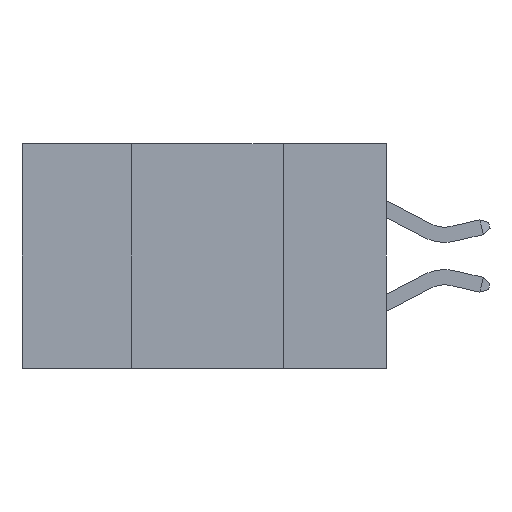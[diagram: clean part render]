
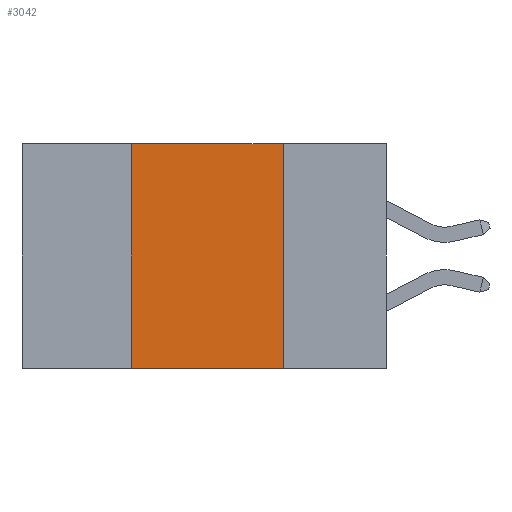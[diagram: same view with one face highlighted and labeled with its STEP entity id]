
A CAD part, left-side view. The second image highlights one B-rep face of the part: STEP entity #3042.
In plain terms, the highlighted planar face has unit normal (-1, 0, 0).
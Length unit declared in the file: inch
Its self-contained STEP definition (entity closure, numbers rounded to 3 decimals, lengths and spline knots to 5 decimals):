
#240 = CARTESIAN_POINT ( 'NONE',  ( 0., 0.17, -0.37 ) ) ;
#822 = ORIENTED_EDGE ( 'NONE', *, *, #5754, .F. ) ;
#826 = LINE ( 'NONE', #240, #7479 ) ;
#827 = DIRECTION ( 'NONE',  ( 1., 0., 0. ) ) ;
#937 = DIRECTION ( 'NONE',  ( 0., 0., 1. ) ) ;
#956 = ORIENTED_EDGE ( 'NONE', *, *, #2574, .F. ) ;
#1021 = VECTOR ( 'NONE', #9868, 39.37008 ) ;
#1038 = ORIENTED_EDGE ( 'NONE', *, *, #1197, .T. ) ;
#1043 = CARTESIAN_POINT ( 'NONE',  ( 0., 0.17, 0. ) ) ;
#1197 = EDGE_CURVE ( 'NONE', #9546, #6426, #2823, .T. ) ;
#1400 = VERTEX_POINT ( 'NONE', #2692 ) ;
#2297 = CARTESIAN_POINT ( 'NONE',  ( 0., 0.6, 0. ) ) ;
#2486 = EDGE_CURVE ( 'NONE', #9546, #1400, #8410, .T. ) ;
#2574 = EDGE_CURVE ( 'NONE', #1400, #7267, #7475, .T. ) ;
#2692 = CARTESIAN_POINT ( 'NONE',  ( 0., 0.42, 0. ) ) ;
#2823 = LINE ( 'NONE', #5846, #9015 ) ;
#3042 = ADVANCED_FACE ( 'NONE', ( #3106 ), #5478, .F. ) ;
#3106 = FACE_OUTER_BOUND ( 'NONE', #3404, .T. ) ;
#3231 = CARTESIAN_POINT ( 'NONE',  ( 0., 0.17, -0.37 ) ) ;
#3244 = VECTOR ( 'NONE', #937, 39.37008 ) ;
#3404 = EDGE_LOOP ( 'NONE', ( #822, #956, #6579, #1038 ) ) ;
#3859 = AXIS2_PLACEMENT_3D ( 'NONE', #2297, #827, #8387 ) ;
#3934 = CARTESIAN_POINT ( 'NONE',  ( 0., 0.42, -0.37 ) ) ;
#4464 = CARTESIAN_POINT ( 'NONE',  ( 0., 0.6, 0. ) ) ;
#4966 = DIRECTION ( 'NONE',  ( 0., -1., 0. ) ) ;
#5478 = PLANE ( 'NONE',  #3859 ) ;
#5754 = EDGE_CURVE ( 'NONE', #7267, #6426, #826, .T. ) ;
#5846 = CARTESIAN_POINT ( 'NONE',  ( 0., 0.6, -0.37 ) ) ;
#6099 = CARTESIAN_POINT ( 'NONE',  ( 0., 0.42, -0.37 ) ) ;
#6426 = VERTEX_POINT ( 'NONE', #3231 ) ;
#6579 = ORIENTED_EDGE ( 'NONE', *, *, #2486, .F. ) ;
#7126 = DIRECTION ( 'NONE',  ( 0., 0., -1. ) ) ;
#7267 = VERTEX_POINT ( 'NONE', #1043 ) ;
#7475 = LINE ( 'NONE', #4464, #1021 ) ;
#7479 = VECTOR ( 'NONE', #7126, 39.37008 ) ;
#8387 = DIRECTION ( 'NONE',  ( 0., 0., -1. ) ) ;
#8410 = LINE ( 'NONE', #6099, #3244 ) ;
#9015 = VECTOR ( 'NONE', #4966, 39.37008 ) ;
#9546 = VERTEX_POINT ( 'NONE', #3934 ) ;
#9868 = DIRECTION ( 'NONE',  ( 0., -1., 0. ) ) ;
